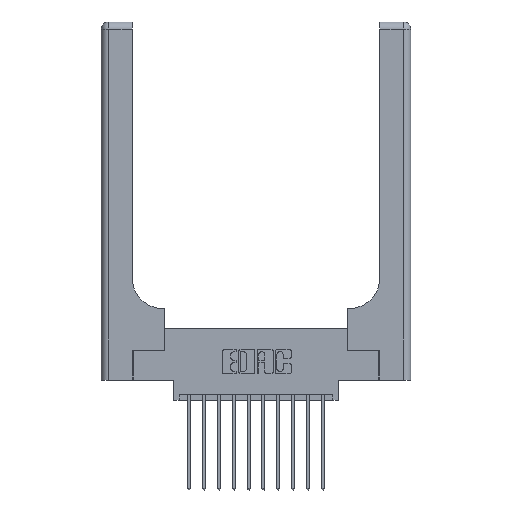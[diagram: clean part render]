
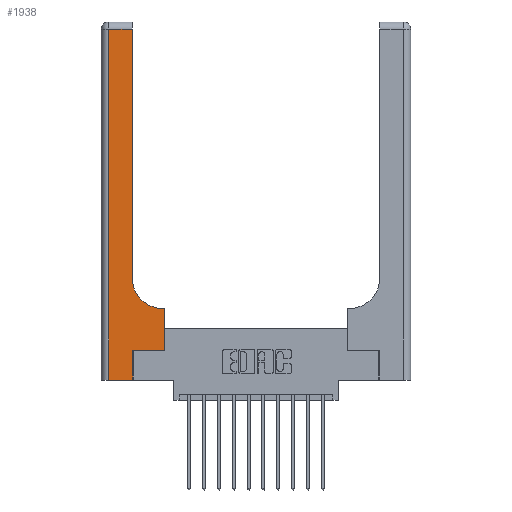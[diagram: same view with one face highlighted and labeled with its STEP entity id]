
A CAD part, top view. The second image highlights one B-rep face of the part: STEP entity #1938.
In plain terms, the highlighted planar face has unit normal (0, 0, 1).
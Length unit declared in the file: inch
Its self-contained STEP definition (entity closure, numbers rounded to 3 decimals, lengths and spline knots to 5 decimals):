
#176 = ORIENTED_EDGE ( 'NONE', *, *, #7128, .T. ) ;
#264 = EDGE_CURVE ( 'NONE', #15217, #14508, #14501, .T. ) ;
#283 = DIRECTION ( 'NONE',  ( 0., 1., 0. ) ) ;
#570 = CARTESIAN_POINT ( 'NONE',  ( 0.528, 0.6, 0.37 ) ) ;
#770 = LINE ( 'NONE', #5980, #11450 ) ;
#1322 = ORIENTED_EDGE ( 'NONE', *, *, #1561, .T. ) ;
#1430 = LINE ( 'NONE', #2539, #13983 ) ;
#1508 = VERTEX_POINT ( 'NONE', #8822 ) ;
#1561 = EDGE_CURVE ( 'NONE', #14508, #11470, #15107, .T. ) ;
#1754 = DIRECTION ( 'NONE',  ( -1., 0., 0. ) ) ;
#1938 = ADVANCED_FACE ( 'NONE', ( #10280 ), #8965, .F. ) ;
#2063 = ORIENTED_EDGE ( 'NONE', *, *, #9872, .T. ) ;
#2162 = LINE ( 'NONE', #10032, #3374 ) ;
#2249 = CARTESIAN_POINT ( 'NONE',  ( 0.528, 0.25, 0.37 ) ) ;
#2297 = DIRECTION ( 'NONE',  ( 1., 0., 0. ) ) ;
#2485 = VECTOR ( 'NONE', #13285, 39.37008 ) ;
#2539 = CARTESIAN_POINT ( 'NONE',  ( 0., 2.94, 0.37 ) ) ;
#2960 = ORIENTED_EDGE ( 'NONE', *, *, #14951, .T. ) ;
#3031 = CARTESIAN_POINT ( 'NONE',  ( 0.26, 0.6, 0.37 ) ) ;
#3374 = VECTOR ( 'NONE', #3438, 39.37008 ) ;
#3438 = DIRECTION ( 'NONE',  ( 0., 1., 0. ) ) ;
#3803 = CARTESIAN_POINT ( 'NONE',  ( 0.265, 0., 0.37 ) ) ;
#3951 = ORIENTED_EDGE ( 'NONE', *, *, #264, .T. ) ;
#4074 = EDGE_CURVE ( 'NONE', #6834, #1508, #1430, .T. ) ;
#4270 = DIRECTION ( 'NONE',  ( 0., 0., -1. ) ) ;
#4294 = CARTESIAN_POINT ( 'NONE',  ( 0.06, 0., 0.37 ) ) ;
#4368 = ORIENTED_EDGE ( 'NONE', *, *, #11551, .T. ) ;
#4547 = ORIENTED_EDGE ( 'NONE', *, *, #9656, .T. ) ;
#5186 = VERTEX_POINT ( 'NONE', #3803 ) ;
#5300 = EDGE_CURVE ( 'NONE', #10679, #15217, #10725, .T. ) ;
#5342 = DIRECTION ( 'NONE',  ( -1., 0., 0. ) ) ;
#5443 = CARTESIAN_POINT ( 'NONE',  ( 0.51, 0.85, 0.37 ) ) ;
#5534 = CARTESIAN_POINT ( 'NONE',  ( 0., 0., 0.37 ) ) ;
#5872 = EDGE_LOOP ( 'NONE', ( #4547, #12892, #2960, #176, #2063, #4368, #8603, #3951, #1322 ) ) ;
#5980 = CARTESIAN_POINT ( 'NONE',  ( 0.265, 0.25, 0.37 ) ) ;
#5993 = CARTESIAN_POINT ( 'NONE',  ( 0.26, 2.94, 0.37 ) ) ;
#6621 = VECTOR ( 'NONE', #283, 39.37008 ) ;
#6670 = VECTOR ( 'NONE', #1754, 39.37008 ) ;
#6682 = CARTESIAN_POINT ( 'NONE',  ( 0.265, 0., 0.37 ) ) ;
#6834 = VERTEX_POINT ( 'NONE', #5993 ) ;
#7128 = EDGE_CURVE ( 'NONE', #16496, #5186, #8308, .T. ) ;
#7136 = DIRECTION ( 'NONE',  ( 1., 0., 0. ) ) ;
#8308 = LINE ( 'NONE', #5534, #11919 ) ;
#8332 = CARTESIAN_POINT ( 'NONE',  ( 0.26, 0.85, 0.37 ) ) ;
#8603 = ORIENTED_EDGE ( 'NONE', *, *, #5300, .T. ) ;
#8822 = CARTESIAN_POINT ( 'NONE',  ( 0.06, 2.94, 0.37 ) ) ;
#8965 = PLANE ( 'NONE',  #11079 ) ;
#9138 = DIRECTION ( 'NONE',  ( 1., 0., 0. ) ) ;
#9656 = EDGE_CURVE ( 'NONE', #11470, #6834, #2162, .T. ) ;
#9872 = EDGE_CURVE ( 'NONE', #5186, #15785, #13145, .T. ) ;
#10032 = CARTESIAN_POINT ( 'NONE',  ( 0.26, 3., 0.37 ) ) ;
#10280 = FACE_OUTER_BOUND ( 'NONE', #5872, .T. ) ;
#10362 = CARTESIAN_POINT ( 'NONE',  ( 0., 3., 0.37 ) ) ;
#10679 = VERTEX_POINT ( 'NONE', #2249 ) ;
#10725 = LINE ( 'NONE', #10814, #2485 ) ;
#10786 = AXIS2_PLACEMENT_3D ( 'NONE', #5443, #4270, #9138 ) ;
#10814 = CARTESIAN_POINT ( 'NONE',  ( 0.528, 0.25, 0.37 ) ) ;
#11079 = AXIS2_PLACEMENT_3D ( 'NONE', #10362, #15447, #5342 ) ;
#11450 = VECTOR ( 'NONE', #2297, 39.37008 ) ;
#11470 = VERTEX_POINT ( 'NONE', #8332 ) ;
#11551 = EDGE_CURVE ( 'NONE', #15785, #10679, #770, .T. ) ;
#11919 = VECTOR ( 'NONE', #7136, 39.37008 ) ;
#12117 = VECTOR ( 'NONE', #13775, 39.37008 ) ;
#12475 = CARTESIAN_POINT ( 'NONE',  ( 0.265, 0.25, 0.37 ) ) ;
#12599 = LINE ( 'NONE', #15118, #12117 ) ;
#12892 = ORIENTED_EDGE ( 'NONE', *, *, #4074, .T. ) ;
#13145 = LINE ( 'NONE', #6682, #6621 ) ;
#13285 = DIRECTION ( 'NONE',  ( 0., 1., 0. ) ) ;
#13324 = CARTESIAN_POINT ( 'NONE',  ( 0.51, 0.6, 0.37 ) ) ;
#13775 = DIRECTION ( 'NONE',  ( 0., -1., 0. ) ) ;
#13983 = VECTOR ( 'NONE', #14267, 39.37008 ) ;
#14267 = DIRECTION ( 'NONE',  ( -1., 0., 0. ) ) ;
#14501 = LINE ( 'NONE', #3031, #6670 ) ;
#14508 = VERTEX_POINT ( 'NONE', #13324 ) ;
#14951 = EDGE_CURVE ( 'NONE', #1508, #16496, #12599, .T. ) ;
#15107 = CIRCLE ( 'NONE', #10786, 0.25 ) ;
#15118 = CARTESIAN_POINT ( 'NONE',  ( 0.06, 3., 0.37 ) ) ;
#15217 = VERTEX_POINT ( 'NONE', #570 ) ;
#15447 = DIRECTION ( 'NONE',  ( 0., 0., -1. ) ) ;
#15785 = VERTEX_POINT ( 'NONE', #12475 ) ;
#16496 = VERTEX_POINT ( 'NONE', #4294 ) ;
